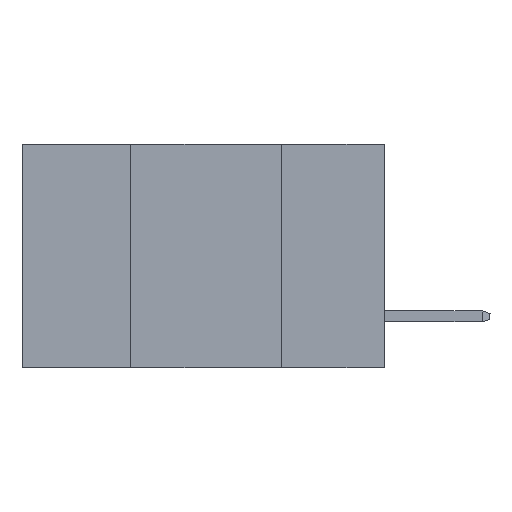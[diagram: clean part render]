
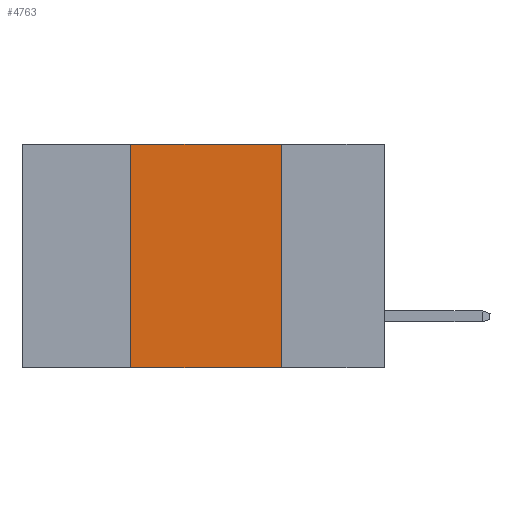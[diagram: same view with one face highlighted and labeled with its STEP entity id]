
A CAD part, left-side view. The second image highlights one B-rep face of the part: STEP entity #4763.
In plain terms, the highlighted planar face has unit normal (-1, 0, 0).
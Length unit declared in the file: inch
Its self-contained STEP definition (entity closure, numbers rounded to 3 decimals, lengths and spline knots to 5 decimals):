
#153 = EDGE_CURVE ( 'NONE', #3521, #8819, #5756, .T. ) ;
#548 = EDGE_CURVE ( 'NONE', #854, #3359, #6532, .T. ) ;
#854 = VERTEX_POINT ( 'NONE', #1137 ) ;
#940 = VECTOR ( 'NONE', #1212, 39.37008 ) ;
#1013 = CARTESIAN_POINT ( 'NONE',  ( 0., 0.42, -0.37 ) ) ;
#1137 = CARTESIAN_POINT ( 'NONE',  ( 0., 0.17, 0. ) ) ;
#1144 = EDGE_CURVE ( 'NONE', #3521, #3359, #6929, .T. ) ;
#1212 = DIRECTION ( 'NONE',  ( 0., -1., 0. ) ) ;
#1226 = LINE ( 'NONE', #3838, #9957 ) ;
#1410 = ORIENTED_EDGE ( 'NONE', *, *, #153, .F. ) ;
#1710 = CARTESIAN_POINT ( 'NONE',  ( 0., 0.17, -0.37 ) ) ;
#2361 = EDGE_CURVE ( 'NONE', #8819, #854, #1226, .T. ) ;
#2717 = DIRECTION ( 'NONE',  ( 0., 0., -1. ) ) ;
#2965 = ORIENTED_EDGE ( 'NONE', *, *, #2361, .F. ) ;
#3052 = VECTOR ( 'NONE', #5182, 39.37008 ) ;
#3176 = CARTESIAN_POINT ( 'NONE',  ( 0., 0.42, 0. ) ) ;
#3359 = VERTEX_POINT ( 'NONE', #1710 ) ;
#3521 = VERTEX_POINT ( 'NONE', #1013 ) ;
#3838 = CARTESIAN_POINT ( 'NONE',  ( 0., 0.6, 0. ) ) ;
#4763 = ADVANCED_FACE ( 'NONE', ( #10076 ), #6026, .F. ) ;
#5042 = CARTESIAN_POINT ( 'NONE',  ( 0., 0.17, -0.37 ) ) ;
#5182 = DIRECTION ( 'NONE',  ( 0., 0., 1. ) ) ;
#5675 = ORIENTED_EDGE ( 'NONE', *, *, #548, .F. ) ;
#5756 = LINE ( 'NONE', #8997, #3052 ) ;
#6026 = PLANE ( 'NONE',  #8123 ) ;
#6080 = DIRECTION ( 'NONE',  ( 0., -1., 0. ) ) ;
#6286 = ORIENTED_EDGE ( 'NONE', *, *, #1144, .T. ) ;
#6532 = LINE ( 'NONE', #5042, #6927 ) ;
#6927 = VECTOR ( 'NONE', #8294, 39.37008 ) ;
#6929 = LINE ( 'NONE', #8474, #940 ) ;
#8123 = AXIS2_PLACEMENT_3D ( 'NONE', #8378, #9967, #2717 ) ;
#8294 = DIRECTION ( 'NONE',  ( 0., 0., -1. ) ) ;
#8378 = CARTESIAN_POINT ( 'NONE',  ( 0., 0.6, 0. ) ) ;
#8474 = CARTESIAN_POINT ( 'NONE',  ( 0., 0.6, -0.37 ) ) ;
#8745 = EDGE_LOOP ( 'NONE', ( #5675, #2965, #1410, #6286 ) ) ;
#8819 = VERTEX_POINT ( 'NONE', #3176 ) ;
#8997 = CARTESIAN_POINT ( 'NONE',  ( 0., 0.42, -0.37 ) ) ;
#9957 = VECTOR ( 'NONE', #6080, 39.37008 ) ;
#9967 = DIRECTION ( 'NONE',  ( 1., 0., 0. ) ) ;
#10076 = FACE_OUTER_BOUND ( 'NONE', #8745, .T. ) ;
